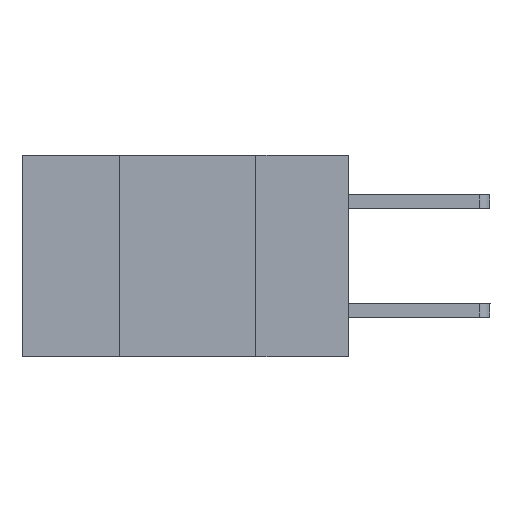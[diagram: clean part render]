
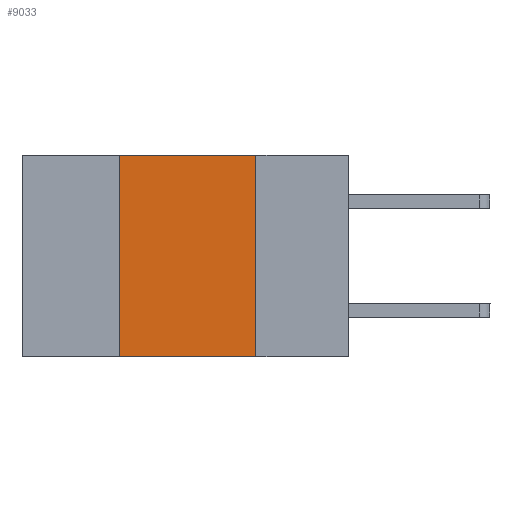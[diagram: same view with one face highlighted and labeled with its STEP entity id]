
A CAD part, left-side view. The second image highlights one B-rep face of the part: STEP entity #9033.
In plain terms, the highlighted planar face has unit normal (-1, 0, 0).
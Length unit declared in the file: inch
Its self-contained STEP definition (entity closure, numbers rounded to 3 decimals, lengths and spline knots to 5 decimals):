
#33 = DIRECTION ( 'NONE',  ( 1., 0., 0. ) ) ;
#833 = LINE ( 'NONE', #9275, #2788 ) ;
#843 = LINE ( 'NONE', #8695, #9502 ) ;
#925 = CARTESIAN_POINT ( 'NONE',  ( 0., 0.6, 0. ) ) ;
#2439 = EDGE_CURVE ( 'NONE', #5861, #4642, #843, .T. ) ;
#2543 = DIRECTION ( 'NONE',  ( 0., 0., -1. ) ) ;
#2788 = VECTOR ( 'NONE', #2543, 39.37008 ) ;
#2870 = DIRECTION ( 'NONE',  ( 0., -1., 0. ) ) ;
#2893 = EDGE_CURVE ( 'NONE', #4046, #4642, #833, .T. ) ;
#3290 = ORIENTED_EDGE ( 'NONE', *, *, #2893, .F. ) ;
#3456 = LINE ( 'NONE', #925, #7680 ) ;
#3540 = CARTESIAN_POINT ( 'NONE',  ( 0., 0.17, -0.37 ) ) ;
#4046 = VERTEX_POINT ( 'NONE', #5195 ) ;
#4084 = ORIENTED_EDGE ( 'NONE', *, *, #2439, .T. ) ;
#4174 = CARTESIAN_POINT ( 'NONE',  ( 0., 0.6, 0. ) ) ;
#4437 = CARTESIAN_POINT ( 'NONE',  ( 0., 0.42, 0. ) ) ;
#4445 = ORIENTED_EDGE ( 'NONE', *, *, #6619, .F. ) ;
#4642 = VERTEX_POINT ( 'NONE', #3540 ) ;
#4770 = EDGE_LOOP ( 'NONE', ( #3290, #4445, #8641, #4084 ) ) ;
#4962 = CARTESIAN_POINT ( 'NONE',  ( 0., 0.42, -0.37 ) ) ;
#5195 = CARTESIAN_POINT ( 'NONE',  ( 0., 0.17, 0. ) ) ;
#5391 = DIRECTION ( 'NONE',  ( 0., 0., 1. ) ) ;
#5861 = VERTEX_POINT ( 'NONE', #4962 ) ;
#5874 = DIRECTION ( 'NONE',  ( 0., 0., -1. ) ) ;
#5927 = DIRECTION ( 'NONE',  ( 0., -1., 0. ) ) ;
#6619 = EDGE_CURVE ( 'NONE', #9232, #4046, #3456, .T. ) ;
#7242 = VECTOR ( 'NONE', #5391, 39.37008 ) ;
#7680 = VECTOR ( 'NONE', #5927, 39.37008 ) ;
#8641 = ORIENTED_EDGE ( 'NONE', *, *, #9960, .F. ) ;
#8695 = CARTESIAN_POINT ( 'NONE',  ( 0., 0.6, -0.37 ) ) ;
#9033 = ADVANCED_FACE ( 'NONE', ( #10520 ), #9217, .F. ) ;
#9217 = PLANE ( 'NONE',  #9477 ) ;
#9232 = VERTEX_POINT ( 'NONE', #4437 ) ;
#9275 = CARTESIAN_POINT ( 'NONE',  ( 0., 0.17, -0.37 ) ) ;
#9477 = AXIS2_PLACEMENT_3D ( 'NONE', #4174, #33, #5874 ) ;
#9502 = VECTOR ( 'NONE', #2870, 39.37008 ) ;
#9584 = CARTESIAN_POINT ( 'NONE',  ( 0., 0.42, -0.37 ) ) ;
#9960 = EDGE_CURVE ( 'NONE', #5861, #9232, #9963, .T. ) ;
#9963 = LINE ( 'NONE', #9584, #7242 ) ;
#10520 = FACE_OUTER_BOUND ( 'NONE', #4770, .T. ) ;
